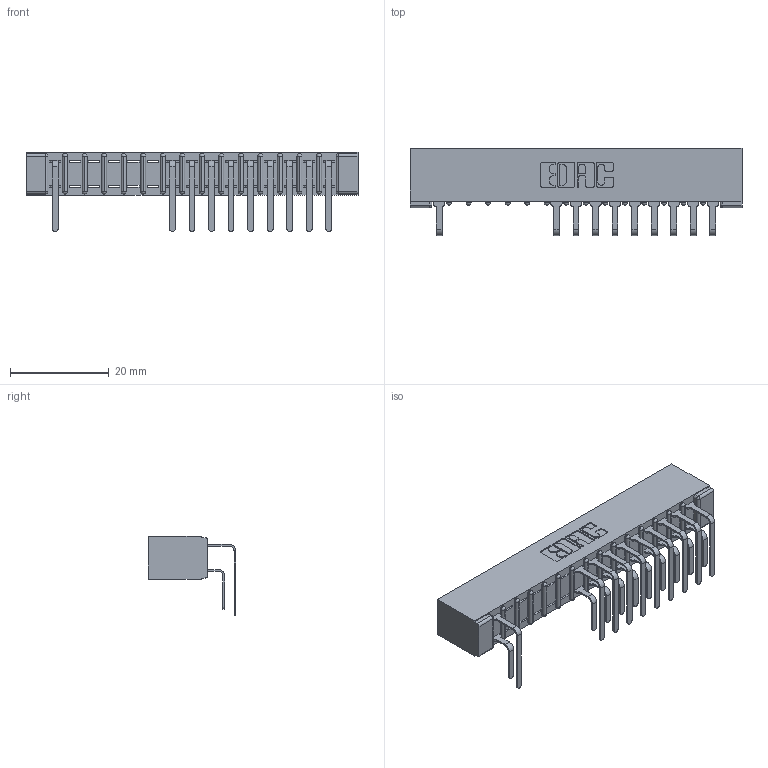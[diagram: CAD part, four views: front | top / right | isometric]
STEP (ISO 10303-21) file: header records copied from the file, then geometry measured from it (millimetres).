
FILE_DESCRIPTION (( 'STEP AP203' ), '1' );
FILE_NAME ('357-015-559-101.STEP', '2018-08-08T01:10:26', ( '' ), ( '' ), 'SwSTEP 2.0', 'SolidWorks 2016', '' );
FILE_SCHEMA (( 'CONFIG_CONTROL_DESIGN' ));
Length unit declared in the file: inch
Products named in the file (4): 307-290-001_559 - 2 (Single); 357-015-559-101; 307 Part_No Mounting Lugs; 307-290-001_558 559 - 1 (Single)
Assembly tree (21 placements, depth 2):
  357-015-559-101
    307 Part_No Mounting Lugs
    307-290-001_558 559 - 1 (Single)  x10
    307-290-001_559 - 2 (Single)  x10
Bounding box: 67.31 x 17.69 x 16.08 mm (x, y, z)
Volume: 4595.9 mm3; surface area: 7957.6 mm2
Topology: 21 solids, 21 shells, 1226 faces, 3459 edges, 2234 vertices
Faces by surface type: plane 786, cylinder 408, sphere 32
Entity records: 17517 total; most frequent: CARTESIAN_POINT 2915, ORIENTED_EDGE 2894, DIRECTION 2855, EDGE_CURVE 1447, VECTOR 1099, LINE 1099, VERTEX_POINT 938, AXIS2_PLACEMENT_3D 878
